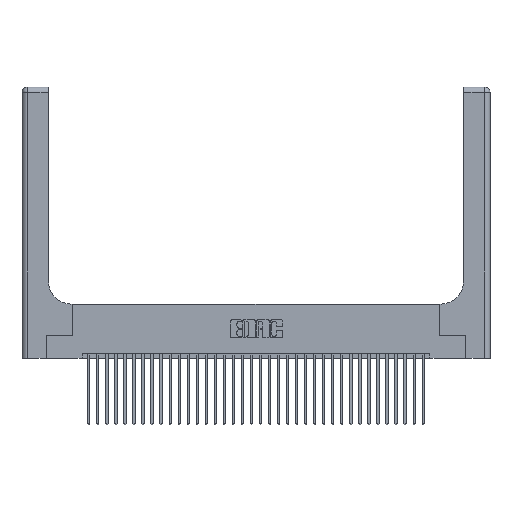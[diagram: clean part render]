
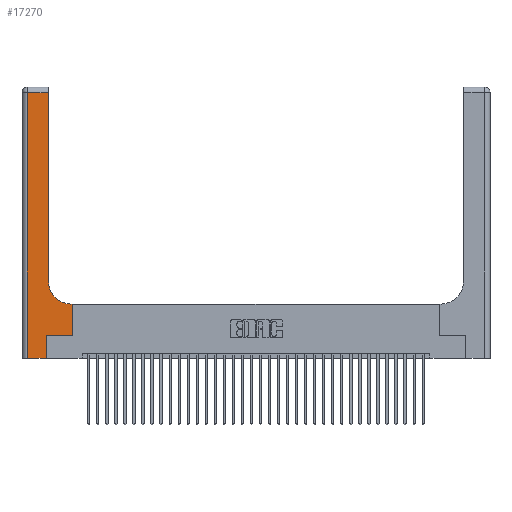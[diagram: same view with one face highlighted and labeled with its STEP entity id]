
A CAD part, top view. The second image highlights one B-rep face of the part: STEP entity #17270.
In plain terms, the highlighted planar face has unit normal (0, 0, 1).
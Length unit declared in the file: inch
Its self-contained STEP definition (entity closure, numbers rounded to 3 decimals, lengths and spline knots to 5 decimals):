
#4 = VERTEX_POINT ( 'NONE', #31909 ) ;
#8 = ORIENTED_EDGE ( 'NONE', *, *, #18792, .T. ) ;
#339 = VECTOR ( 'NONE', #28051, 39.37008 ) ;
#628 = DIRECTION ( 'NONE',  ( 0., 0., -1. ) ) ;
#974 = AXIS2_PLACEMENT_3D ( 'NONE', #32923, #24907, #8367 ) ;
#980 = VECTOR ( 'NONE', #9164, 39.37008 ) ;
#2281 = EDGE_CURVE ( 'NONE', #19533, #4, #15835, .T. ) ;
#2530 = EDGE_CURVE ( 'NONE', #13058, #31480, #3155, .T. ) ;
#2544 = EDGE_LOOP ( 'NONE', ( #7469, #32837, #18079, #14729, #27571, #8, #6188, #9156, #23463 ) ) ;
#3155 = LINE ( 'NONE', #26843, #29895 ) ;
#3214 = LINE ( 'NONE', #9981, #31625 ) ;
#3735 = EDGE_CURVE ( 'NONE', #12339, #16964, #12679, .T. ) ;
#4393 = VERTEX_POINT ( 'NONE', #12676 ) ;
#5258 = VERTEX_POINT ( 'NONE', #12386 ) ;
#5581 = CARTESIAN_POINT ( 'NONE',  ( 0.06, 0., 0.37 ) ) ;
#6098 = LINE ( 'NONE', #12506, #27269 ) ;
#6188 = ORIENTED_EDGE ( 'NONE', *, *, #2281, .T. ) ;
#6237 = EDGE_CURVE ( 'NONE', #4393, #12339, #15181, .T. ) ;
#7439 = VERTEX_POINT ( 'NONE', #17579 ) ;
#7469 = ORIENTED_EDGE ( 'NONE', *, *, #23807, .T. ) ;
#8027 = CARTESIAN_POINT ( 'NONE',  ( 0.269, 0., 0.37 ) ) ;
#8367 = DIRECTION ( 'NONE',  ( -1., 0., 0. ) ) ;
#8554 = CARTESIAN_POINT ( 'NONE',  ( 0.2915, 0.6, 0.37 ) ) ;
#9156 = ORIENTED_EDGE ( 'NONE', *, *, #31328, .T. ) ;
#9164 = DIRECTION ( 'NONE',  ( 0., 1., 0. ) ) ;
#9328 = AXIS2_PLACEMENT_3D ( 'NONE', #17352, #628, #20085 ) ;
#9922 = DIRECTION ( 'NONE',  ( 0., 1., 0. ) ) ;
#9981 = CARTESIAN_POINT ( 'NONE',  ( 0.269, 0.25, 0.37 ) ) ;
#10618 = CARTESIAN_POINT ( 'NONE',  ( 0.06, 2.94, 0.37 ) ) ;
#11586 = CARTESIAN_POINT ( 'NONE',  ( 0., 2.94, 0.37 ) ) ;
#12339 = VERTEX_POINT ( 'NONE', #10618 ) ;
#12386 = CARTESIAN_POINT ( 'NONE',  ( 0.2915, 0.85, 0.37 ) ) ;
#12506 = CARTESIAN_POINT ( 'NONE',  ( 0., 0., 0.37 ) ) ;
#12676 = CARTESIAN_POINT ( 'NONE',  ( 0.2915, 2.94, 0.37 ) ) ;
#12679 = LINE ( 'NONE', #12845, #33601 ) ;
#12845 = CARTESIAN_POINT ( 'NONE',  ( 0.06, 3., 0.37 ) ) ;
#13058 = VERTEX_POINT ( 'NONE', #8027 ) ;
#13150 = DIRECTION ( 'NONE',  ( 0., 1., 0. ) ) ;
#13687 = VECTOR ( 'NONE', #9922, 39.37008 ) ;
#14729 = ORIENTED_EDGE ( 'NONE', *, *, #30335, .T. ) ;
#15181 = LINE ( 'NONE', #11586, #339 ) ;
#15835 = LINE ( 'NONE', #22917, #980 ) ;
#16964 = VERTEX_POINT ( 'NONE', #5581 ) ;
#17270 = ADVANCED_FACE ( 'NONE', ( #35514 ), #19397, .F. ) ;
#17352 = CARTESIAN_POINT ( 'NONE',  ( 0.5415, 0.85, 0.37 ) ) ;
#17579 = CARTESIAN_POINT ( 'NONE',  ( 0.5415, 0.6, 0.37 ) ) ;
#18079 = ORIENTED_EDGE ( 'NONE', *, *, #3735, .T. ) ;
#18349 = DIRECTION ( 'NONE',  ( 1., 0., 0. ) ) ;
#18792 = EDGE_CURVE ( 'NONE', #31480, #19533, #3214, .T. ) ;
#19397 = PLANE ( 'NONE',  #974 ) ;
#19533 = VERTEX_POINT ( 'NONE', #23924 ) ;
#20085 = DIRECTION ( 'NONE',  ( 1., 0., 0. ) ) ;
#21010 = EDGE_CURVE ( 'NONE', #7439, #5258, #28159, .T. ) ;
#21012 = LINE ( 'NONE', #23666, #13687 ) ;
#22917 = CARTESIAN_POINT ( 'NONE',  ( 0.5585, 0.25, 0.37 ) ) ;
#23463 = ORIENTED_EDGE ( 'NONE', *, *, #21010, .T. ) ;
#23666 = CARTESIAN_POINT ( 'NONE',  ( 0.2915, 3., 0.37 ) ) ;
#23807 = EDGE_CURVE ( 'NONE', #5258, #4393, #21012, .T. ) ;
#23924 = CARTESIAN_POINT ( 'NONE',  ( 0.5585, 0.25, 0.37 ) ) ;
#24907 = DIRECTION ( 'NONE',  ( 0., 0., -1. ) ) ;
#25090 = DIRECTION ( 'NONE',  ( -1., 0., 0. ) ) ;
#25504 = LINE ( 'NONE', #8554, #31826 ) ;
#26843 = CARTESIAN_POINT ( 'NONE',  ( 0.269, 0., 0.37 ) ) ;
#27269 = VECTOR ( 'NONE', #31641, 39.37008 ) ;
#27571 = ORIENTED_EDGE ( 'NONE', *, *, #2530, .T. ) ;
#28051 = DIRECTION ( 'NONE',  ( -1., 0., 0. ) ) ;
#28159 = CIRCLE ( 'NONE', #9328, 0.25 ) ;
#28269 = CARTESIAN_POINT ( 'NONE',  ( 0.269, 0.25, 0.37 ) ) ;
#29895 = VECTOR ( 'NONE', #13150, 39.37008 ) ;
#30335 = EDGE_CURVE ( 'NONE', #16964, #13058, #6098, .T. ) ;
#31328 = EDGE_CURVE ( 'NONE', #4, #7439, #25504, .T. ) ;
#31480 = VERTEX_POINT ( 'NONE', #28269 ) ;
#31625 = VECTOR ( 'NONE', #18349, 39.37008 ) ;
#31641 = DIRECTION ( 'NONE',  ( 1., 0., 0. ) ) ;
#31826 = VECTOR ( 'NONE', #25090, 39.37008 ) ;
#31909 = CARTESIAN_POINT ( 'NONE',  ( 0.5585, 0.6, 0.37 ) ) ;
#32837 = ORIENTED_EDGE ( 'NONE', *, *, #6237, .T. ) ;
#32923 = CARTESIAN_POINT ( 'NONE',  ( 0., 3., 0.37 ) ) ;
#33601 = VECTOR ( 'NONE', #34646, 39.37008 ) ;
#34646 = DIRECTION ( 'NONE',  ( 0., -1., 0. ) ) ;
#35514 = FACE_OUTER_BOUND ( 'NONE', #2544, .T. ) ;
